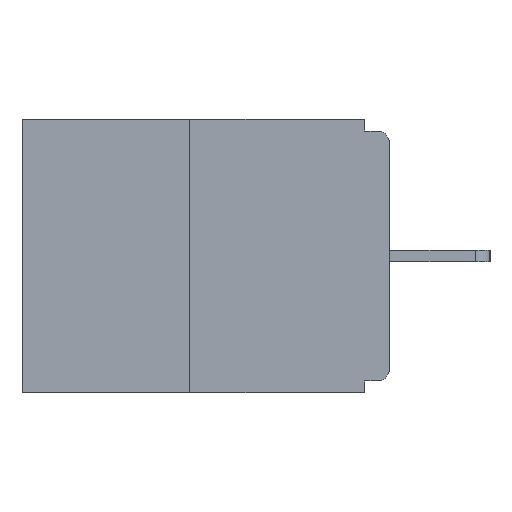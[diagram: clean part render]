
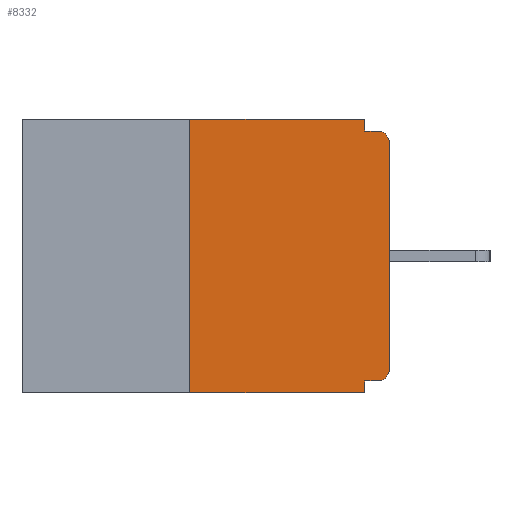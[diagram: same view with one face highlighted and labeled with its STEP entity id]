
A CAD part, left-side view. The second image highlights one B-rep face of the part: STEP entity #8332.
In plain terms, the highlighted planar face has unit normal (-1, 0, 0).
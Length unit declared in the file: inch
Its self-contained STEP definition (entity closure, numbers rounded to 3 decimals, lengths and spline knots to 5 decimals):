
#89 = FACE_OUTER_BOUND ( 'NONE', #14117, .T. ) ;
#377 = LINE ( 'NONE', #7818, #6189 ) ;
#432 = EDGE_CURVE ( 'NONE', #8432, #2321, #895, .T. ) ;
#590 = CARTESIAN_POINT ( 'NONE',  ( 0., 0.015, -0.328 ) ) ;
#769 = DIRECTION ( 'NONE',  ( 0., 0., -1. ) ) ;
#771 = DIRECTION ( 'NONE',  ( 0., 0., 1. ) ) ;
#781 = ORIENTED_EDGE ( 'NONE', *, *, #13928, .F. ) ;
#845 = VERTEX_POINT ( 'NONE', #2536 ) ;
#895 = CIRCLE ( 'NONE', #7639, 0.015 ) ;
#1070 = CARTESIAN_POINT ( 'NONE',  ( 0., 0., -0.313 ) ) ;
#1099 = LINE ( 'NONE', #1940, #8113 ) ;
#1149 = VECTOR ( 'NONE', #8860, 39.37008 ) ;
#1187 = AXIS2_PLACEMENT_3D ( 'NONE', #4830, #8185, #8086 ) ;
#1216 = VERTEX_POINT ( 'NONE', #6662 ) ;
#1425 = CARTESIAN_POINT ( 'NONE',  ( 0., 0.25, -0.343 ) ) ;
#1789 = ORIENTED_EDGE ( 'NONE', *, *, #9272, .F. ) ;
#1798 = EDGE_CURVE ( 'NONE', #13436, #2321, #14558, .T. ) ;
#1940 = CARTESIAN_POINT ( 'NONE',  ( 0., 0., -0.328 ) ) ;
#2185 = CARTESIAN_POINT ( 'NONE',  ( 0., 0.015, -0.313 ) ) ;
#2203 = PLANE ( 'NONE',  #1187 ) ;
#2321 = VERTEX_POINT ( 'NONE', #5031 ) ;
#2353 = ORIENTED_EDGE ( 'NONE', *, *, #5748, .F. ) ;
#2536 = CARTESIAN_POINT ( 'NONE',  ( 0., 0.031, 0. ) ) ;
#2613 = CARTESIAN_POINT ( 'NONE',  ( 0., 0.46, 0. ) ) ;
#3318 = DIRECTION ( 'NONE',  ( 0., 0., -1. ) ) ;
#3830 = VERTEX_POINT ( 'NONE', #10442 ) ;
#4065 = CARTESIAN_POINT ( 'NONE',  ( 0., 0.015, -0.03 ) ) ;
#4148 = LINE ( 'NONE', #11099, #12258 ) ;
#4149 = CARTESIAN_POINT ( 'NONE',  ( 0., 0.25, 0. ) ) ;
#4197 = AXIS2_PLACEMENT_3D ( 'NONE', #2185, #5650, #3318 ) ;
#4217 = VERTEX_POINT ( 'NONE', #1070 ) ;
#4830 = CARTESIAN_POINT ( 'NONE',  ( 0., 0.46, 0. ) ) ;
#5031 = CARTESIAN_POINT ( 'NONE',  ( 0., 0.015, -0.015 ) ) ;
#5091 = ORIENTED_EDGE ( 'NONE', *, *, #10359, .T. ) ;
#5209 = ORIENTED_EDGE ( 'NONE', *, *, #432, .T. ) ;
#5642 = ORIENTED_EDGE ( 'NONE', *, *, #8810, .T. ) ;
#5650 = DIRECTION ( 'NONE',  ( -1., 0., 0. ) ) ;
#5736 = CARTESIAN_POINT ( 'NONE',  ( 0., 0.031, -0.015 ) ) ;
#5748 = EDGE_CURVE ( 'NONE', #845, #13436, #9987, .T. ) ;
#5891 = CIRCLE ( 'NONE', #4197, 0.015 ) ;
#6119 = DIRECTION ( 'NONE',  ( 0., -1., 0. ) ) ;
#6189 = VECTOR ( 'NONE', #771, 39.37008 ) ;
#6322 = CARTESIAN_POINT ( 'NONE',  ( 0., 0.031, 0. ) ) ;
#6447 = VECTOR ( 'NONE', #769, 39.37008 ) ;
#6662 = CARTESIAN_POINT ( 'NONE',  ( 0., 0.031, -0.343 ) ) ;
#6693 = CARTESIAN_POINT ( 'NONE',  ( 0., 0., -0.015 ) ) ;
#7096 = VECTOR ( 'NONE', #6119, 39.37008 ) ;
#7404 = VERTEX_POINT ( 'NONE', #590 ) ;
#7639 = AXIS2_PLACEMENT_3D ( 'NONE', #4065, #9693, #14027 ) ;
#7809 = VECTOR ( 'NONE', #8509, 39.37008 ) ;
#7818 = CARTESIAN_POINT ( 'NONE',  ( 0., 0., 0. ) ) ;
#8001 = ORIENTED_EDGE ( 'NONE', *, *, #14341, .F. ) ;
#8086 = DIRECTION ( 'NONE',  ( 0., 0., -1. ) ) ;
#8113 = VECTOR ( 'NONE', #12038, 39.37008 ) ;
#8185 = DIRECTION ( 'NONE',  ( 1., 0., 0. ) ) ;
#8332 = ADVANCED_FACE ( 'NONE', ( #89 ), #2203, .F. ) ;
#8432 = VERTEX_POINT ( 'NONE', #11841 ) ;
#8509 = DIRECTION ( 'NONE',  ( 0., 0., -1. ) ) ;
#8810 = EDGE_CURVE ( 'NONE', #12060, #1216, #9397, .T. ) ;
#8860 = DIRECTION ( 'NONE',  ( 0., -1., 0. ) ) ;
#8898 = LINE ( 'NONE', #13065, #7809 ) ;
#9050 = EDGE_CURVE ( 'NONE', #7404, #4217, #5891, .T. ) ;
#9272 = EDGE_CURVE ( 'NONE', #10405, #845, #10307, .T. ) ;
#9397 = LINE ( 'NONE', #13423, #11531 ) ;
#9693 = DIRECTION ( 'NONE',  ( -1., 0., 0. ) ) ;
#9872 = DIRECTION ( 'NONE',  ( 0., 0., 1. ) ) ;
#9987 = LINE ( 'NONE', #6322, #6447 ) ;
#10030 = EDGE_CURVE ( 'NONE', #7404, #3830, #1099, .T. ) ;
#10073 = DIRECTION ( 'NONE',  ( 0., -1., 0. ) ) ;
#10307 = LINE ( 'NONE', #2613, #7096 ) ;
#10359 = EDGE_CURVE ( 'NONE', #4217, #8432, #377, .T. ) ;
#10405 = VERTEX_POINT ( 'NONE', #4149 ) ;
#10442 = CARTESIAN_POINT ( 'NONE',  ( 0., 0.031, -0.328 ) ) ;
#11099 = CARTESIAN_POINT ( 'NONE',  ( 0., 0.25, 0. ) ) ;
#11377 = ORIENTED_EDGE ( 'NONE', *, *, #1798, .F. ) ;
#11531 = VECTOR ( 'NONE', #10073, 39.37008 ) ;
#11841 = CARTESIAN_POINT ( 'NONE',  ( 0., 0., -0.03 ) ) ;
#12038 = DIRECTION ( 'NONE',  ( 0., 1., 0. ) ) ;
#12060 = VERTEX_POINT ( 'NONE', #1425 ) ;
#12258 = VECTOR ( 'NONE', #9872, 39.37008 ) ;
#13065 = CARTESIAN_POINT ( 'NONE',  ( 0., 0.031, -0.343 ) ) ;
#13423 = CARTESIAN_POINT ( 'NONE',  ( 0., 0.46, -0.343 ) ) ;
#13436 = VERTEX_POINT ( 'NONE', #5736 ) ;
#13881 = ORIENTED_EDGE ( 'NONE', *, *, #9050, .T. ) ;
#13928 = EDGE_CURVE ( 'NONE', #12060, #10405, #4148, .T. ) ;
#14027 = DIRECTION ( 'NONE',  ( 0., 0., -1. ) ) ;
#14117 = EDGE_LOOP ( 'NONE', ( #1789, #781, #5642, #8001, #14135, #13881, #5091, #5209, #11377, #2353 ) ) ;
#14135 = ORIENTED_EDGE ( 'NONE', *, *, #10030, .F. ) ;
#14341 = EDGE_CURVE ( 'NONE', #3830, #1216, #8898, .T. ) ;
#14558 = LINE ( 'NONE', #6693, #1149 ) ;
